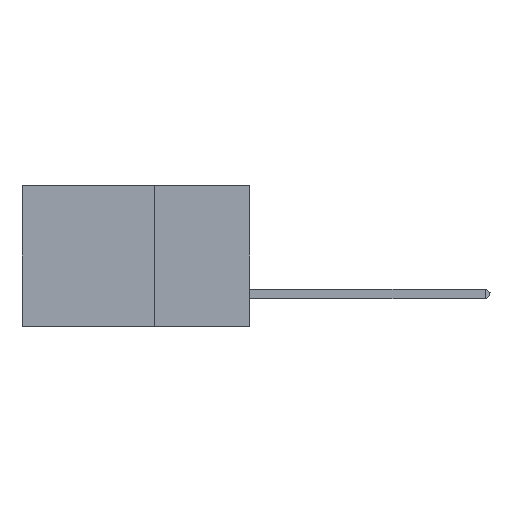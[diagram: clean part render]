
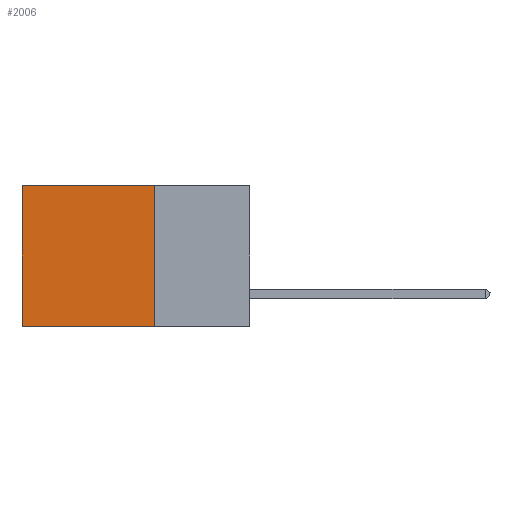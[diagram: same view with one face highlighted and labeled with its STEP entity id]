
A CAD part, left-side view. The second image highlights one B-rep face of the part: STEP entity #2006.
In plain terms, the highlighted planar face has unit normal (-1, 0, 0).
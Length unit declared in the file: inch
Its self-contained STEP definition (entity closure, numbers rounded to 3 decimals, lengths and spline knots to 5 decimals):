
#329 = LINE ( 'NONE', #2281, #835 ) ;
#835 = VECTOR ( 'NONE', #9112, 39.37008 ) ;
#848 = LINE ( 'NONE', #10005, #2468 ) ;
#1056 = FACE_OUTER_BOUND ( 'NONE', #8017, .T. ) ;
#1171 = DIRECTION ( 'NONE',  ( 1., 0., 0. ) ) ;
#2006 = ADVANCED_FACE ( 'NONE', ( #1056 ), #7028, .F. ) ;
#2047 = VERTEX_POINT ( 'NONE', #6218 ) ;
#2281 = CARTESIAN_POINT ( 'NONE',  ( 0.2875, 0.25, 0. ) ) ;
#2468 = VECTOR ( 'NONE', #7783, 39.37008 ) ;
#2668 = ORIENTED_EDGE ( 'NONE', *, *, #10531, .F. ) ;
#2697 = EDGE_CURVE ( 'NONE', #6951, #6154, #848, .T. ) ;
#2913 = EDGE_CURVE ( 'NONE', #6951, #2047, #329, .T. ) ;
#3055 = VECTOR ( 'NONE', #7611, 39.37008 ) ;
#3635 = CARTESIAN_POINT ( 'NONE',  ( 0.2875, 0.6, -0.37 ) ) ;
#3966 = CARTESIAN_POINT ( 'NONE',  ( 0.2875, 0.6, 0. ) ) ;
#4351 = VECTOR ( 'NONE', #14167, 39.37008 ) ;
#4539 = CARTESIAN_POINT ( 'NONE',  ( 0.2875, 0.25, -0.37 ) ) ;
#4633 = CARTESIAN_POINT ( 'NONE',  ( 0.2875, 0.25, 0. ) ) ;
#4842 = LINE ( 'NONE', #8670, #3055 ) ;
#6154 = VERTEX_POINT ( 'NONE', #4539 ) ;
#6218 = CARTESIAN_POINT ( 'NONE',  ( 0.2875, 0.6, 0. ) ) ;
#6603 = AXIS2_PLACEMENT_3D ( 'NONE', #4633, #1171, #11504 ) ;
#6741 = ORIENTED_EDGE ( 'NONE', *, *, #7329, .T. ) ;
#6951 = VERTEX_POINT ( 'NONE', #9427 ) ;
#7028 = PLANE ( 'NONE',  #6603 ) ;
#7329 = EDGE_CURVE ( 'NONE', #2047, #8936, #10838, .T. ) ;
#7611 = DIRECTION ( 'NONE',  ( 0., 1., 0. ) ) ;
#7783 = DIRECTION ( 'NONE',  ( 0., 0., -1. ) ) ;
#8017 = EDGE_LOOP ( 'NONE', ( #6741, #2668, #12528, #9888 ) ) ;
#8670 = CARTESIAN_POINT ( 'NONE',  ( 0.2875, 0.25, -0.37 ) ) ;
#8936 = VERTEX_POINT ( 'NONE', #3635 ) ;
#9112 = DIRECTION ( 'NONE',  ( 0., 1., 0. ) ) ;
#9427 = CARTESIAN_POINT ( 'NONE',  ( 0.2875, 0.25, 0. ) ) ;
#9888 = ORIENTED_EDGE ( 'NONE', *, *, #2913, .T. ) ;
#10005 = CARTESIAN_POINT ( 'NONE',  ( 0.2875, 0.25, 0. ) ) ;
#10531 = EDGE_CURVE ( 'NONE', #6154, #8936, #4842, .T. ) ;
#10838 = LINE ( 'NONE', #3966, #4351 ) ;
#11504 = DIRECTION ( 'NONE',  ( 0., 0., -1. ) ) ;
#12528 = ORIENTED_EDGE ( 'NONE', *, *, #2697, .F. ) ;
#14167 = DIRECTION ( 'NONE',  ( 0., 0., -1. ) ) ;
